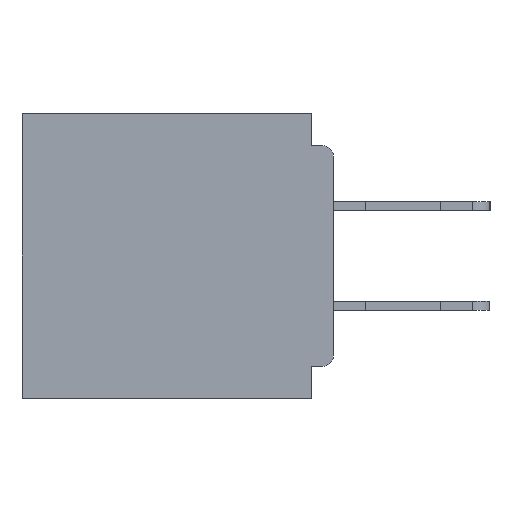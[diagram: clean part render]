
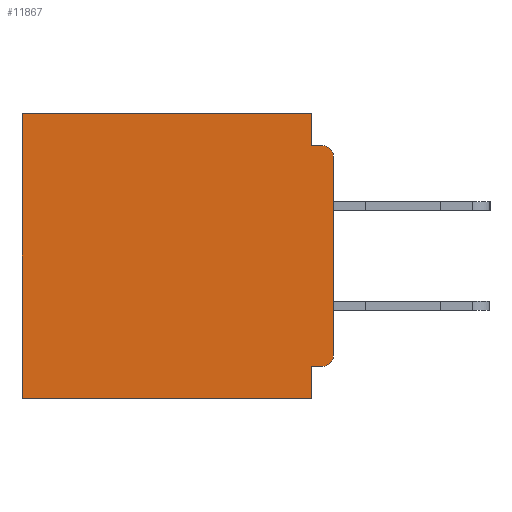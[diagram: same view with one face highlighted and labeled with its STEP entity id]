
A CAD part, left-side view. The second image highlights one B-rep face of the part: STEP entity #11867.
In plain terms, the highlighted planar face has unit normal (-1, 0, 0).
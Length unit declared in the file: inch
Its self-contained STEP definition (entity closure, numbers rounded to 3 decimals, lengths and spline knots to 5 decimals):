
#672 = ORIENTED_EDGE ( 'NONE', *, *, #37230, .F. ) ;
#784 = VERTEX_POINT ( 'NONE', #31434 ) ;
#930 = VERTEX_POINT ( 'NONE', #37291 ) ;
#1164 = VERTEX_POINT ( 'NONE', #12018 ) ;
#1358 = VECTOR ( 'NONE', #18343, 39.37008 ) ;
#1465 = VECTOR ( 'NONE', #36294, 39.37008 ) ;
#2248 = LINE ( 'NONE', #10486, #18262 ) ;
#3233 = DIRECTION ( 'NONE',  ( 0., 0., -1. ) ) ;
#4542 = CARTESIAN_POINT ( 'NONE',  ( 0.3, 0., -0.4 ) ) ;
#5090 = LINE ( 'NONE', #4542, #40249 ) ;
#5285 = VECTOR ( 'NONE', #38404, 39.37008 ) ;
#5403 = VERTEX_POINT ( 'NONE', #32921 ) ;
#6015 = ORIENTED_EDGE ( 'NONE', *, *, #12643, .F. ) ;
#7013 = DIRECTION ( 'NONE',  ( 0., 0., -1. ) ) ;
#7577 = EDGE_CURVE ( 'NONE', #28290, #41258, #39945, .T. ) ;
#8863 = EDGE_CURVE ( 'NONE', #5403, #37062, #10589, .T. ) ;
#10486 = CARTESIAN_POINT ( 'NONE',  ( 0.3, 0., -0.4 ) ) ;
#10589 = LINE ( 'NONE', #22592, #1465 ) ;
#10696 = VECTOR ( 'NONE', #7013, 39.37008 ) ;
#11867 = ADVANCED_FACE ( 'NONE', ( #40582 ), #20212, .F. ) ;
#12018 = CARTESIAN_POINT ( 'NONE',  ( 0.3, 0.031, -0.4 ) ) ;
#12532 = ORIENTED_EDGE ( 'NONE', *, *, #21256, .T. ) ;
#12643 = EDGE_CURVE ( 'NONE', #1164, #40459, #2248, .T. ) ;
#14274 = VECTOR ( 'NONE', #30340, 39.37008 ) ;
#14432 = LINE ( 'NONE', #35004, #5285 ) ;
#15463 = CARTESIAN_POINT ( 'NONE',  ( 0.3, 0.015, -0.34 ) ) ;
#16036 = CARTESIAN_POINT ( 'NONE',  ( 0.3, 0., -0.06 ) ) ;
#17594 = EDGE_CURVE ( 'NONE', #930, #40459, #40324, .T. ) ;
#17944 = ORIENTED_EDGE ( 'NONE', *, *, #8863, .F. ) ;
#18262 = VECTOR ( 'NONE', #41078, 39.37008 ) ;
#18343 = DIRECTION ( 'NONE',  ( 0., -1., 0. ) ) ;
#18627 = DIRECTION ( 'NONE',  ( -1., 0., 0. ) ) ;
#18840 = DIRECTION ( 'NONE',  ( 0., 0., -1. ) ) ;
#19536 = AXIS2_PLACEMENT_3D ( 'NONE', #44024, #23630, #3233 ) ;
#19692 = LINE ( 'NONE', #20548, #10696 ) ;
#19780 = AXIS2_PLACEMENT_3D ( 'NONE', #38984, #18627, #42399 ) ;
#20212 = PLANE ( 'NONE',  #19536 ) ;
#20548 = CARTESIAN_POINT ( 'NONE',  ( 0.3, 0.031, -0.4 ) ) ;
#21256 = EDGE_CURVE ( 'NONE', #40907, #28650, #27483, .T. ) ;
#21858 = EDGE_CURVE ( 'NONE', #40907, #41258, #5090, .T. ) ;
#22592 = CARTESIAN_POINT ( 'NONE',  ( 0.3, 0.031, 0. ) ) ;
#23529 = CARTESIAN_POINT ( 'NONE',  ( 0.3, 0., 0. ) ) ;
#23630 = DIRECTION ( 'NONE',  ( 1., 0., 0. ) ) ;
#24112 = ORIENTED_EDGE ( 'NONE', *, *, #26902, .T. ) ;
#26902 = EDGE_CURVE ( 'NONE', #5403, #930, #33336, .T. ) ;
#27207 = EDGE_CURVE ( 'NONE', #37062, #28650, #37597, .T. ) ;
#27483 = CIRCLE ( 'NONE', #19780, 0.015 ) ;
#28010 = CARTESIAN_POINT ( 'NONE',  ( 0.3, 0.437, -0.4 ) ) ;
#28290 = VERTEX_POINT ( 'NONE', #30829 ) ;
#28650 = VERTEX_POINT ( 'NONE', #43039 ) ;
#29353 = ORIENTED_EDGE ( 'NONE', *, *, #21858, .F. ) ;
#29940 = ORIENTED_EDGE ( 'NONE', *, *, #37066, .F. ) ;
#30340 = DIRECTION ( 'NONE',  ( 0., 1., 0. ) ) ;
#30829 = CARTESIAN_POINT ( 'NONE',  ( 0.3, 0.015, -0.355 ) ) ;
#31239 = VECTOR ( 'NONE', #34887, 39.37008 ) ;
#31434 = CARTESIAN_POINT ( 'NONE',  ( 0.3, 0.031, -0.355 ) ) ;
#31758 = DIRECTION ( 'NONE',  ( 0., 0., -1. ) ) ;
#32921 = CARTESIAN_POINT ( 'NONE',  ( 0.3, 0.031, 0. ) ) ;
#33336 = LINE ( 'NONE', #23529, #14274 ) ;
#34887 = DIRECTION ( 'NONE',  ( 0., 0., -1. ) ) ;
#35004 = CARTESIAN_POINT ( 'NONE',  ( 0.3, 0., -0.355 ) ) ;
#35847 = ORIENTED_EDGE ( 'NONE', *, *, #7577, .T. ) ;
#36294 = DIRECTION ( 'NONE',  ( 0., 0., -1. ) ) ;
#36358 = ORIENTED_EDGE ( 'NONE', *, *, #27207, .F. ) ;
#37062 = VERTEX_POINT ( 'NONE', #40940 ) ;
#37066 = EDGE_CURVE ( 'NONE', #784, #1164, #19692, .T. ) ;
#37230 = EDGE_CURVE ( 'NONE', #28290, #784, #14432, .T. ) ;
#37291 = CARTESIAN_POINT ( 'NONE',  ( 0.3, 0.437, 0. ) ) ;
#37596 = CARTESIAN_POINT ( 'NONE',  ( 0.3, 0.437, -0.4 ) ) ;
#37597 = LINE ( 'NONE', #38707, #1358 ) ;
#38404 = DIRECTION ( 'NONE',  ( 0., 1., 0. ) ) ;
#38590 = EDGE_LOOP ( 'NONE', ( #29353, #12532, #36358, #17944, #24112, #40060, #6015, #29940, #672, #35847 ) ) ;
#38707 = CARTESIAN_POINT ( 'NONE',  ( 0.3, 0., -0.045 ) ) ;
#38984 = CARTESIAN_POINT ( 'NONE',  ( 0.3, 0.015, -0.06 ) ) ;
#39216 = DIRECTION ( 'NONE',  ( -1., 0., 0. ) ) ;
#39459 = AXIS2_PLACEMENT_3D ( 'NONE', #15463, #39216, #18840 ) ;
#39945 = CIRCLE ( 'NONE', #39459, 0.015 ) ;
#40060 = ORIENTED_EDGE ( 'NONE', *, *, #17594, .T. ) ;
#40249 = VECTOR ( 'NONE', #31758, 39.37008 ) ;
#40324 = LINE ( 'NONE', #28010, #31239 ) ;
#40459 = VERTEX_POINT ( 'NONE', #37596 ) ;
#40582 = FACE_OUTER_BOUND ( 'NONE', #38590, .T. ) ;
#40907 = VERTEX_POINT ( 'NONE', #16036 ) ;
#40940 = CARTESIAN_POINT ( 'NONE',  ( 0.3, 0.031, -0.045 ) ) ;
#41078 = DIRECTION ( 'NONE',  ( 0., 1., 0. ) ) ;
#41258 = VERTEX_POINT ( 'NONE', #41846 ) ;
#41846 = CARTESIAN_POINT ( 'NONE',  ( 0.3, 0., -0.34 ) ) ;
#42399 = DIRECTION ( 'NONE',  ( 0., 0., -1. ) ) ;
#43039 = CARTESIAN_POINT ( 'NONE',  ( 0.3, 0.015, -0.045 ) ) ;
#44024 = CARTESIAN_POINT ( 'NONE',  ( 0.3, 0., -0.4 ) ) ;
